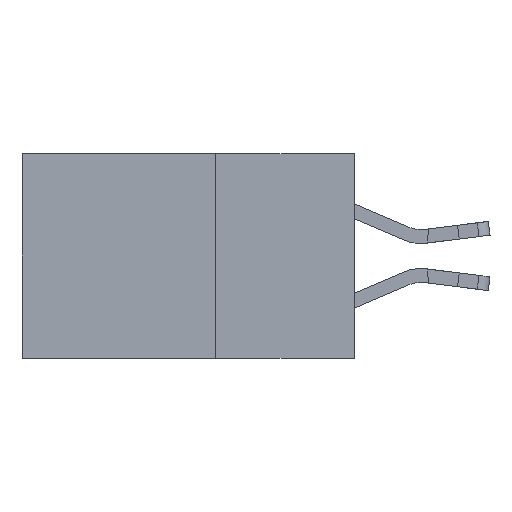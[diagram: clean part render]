
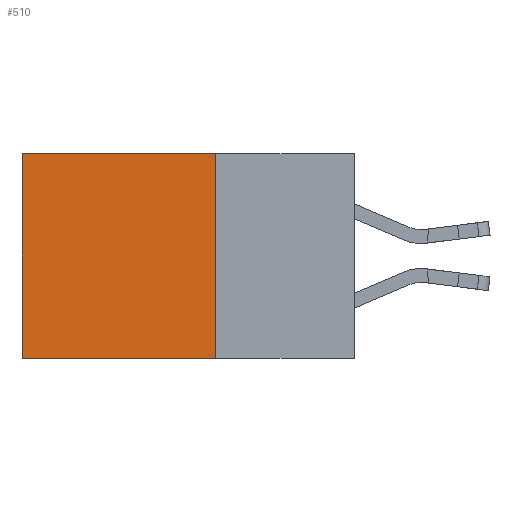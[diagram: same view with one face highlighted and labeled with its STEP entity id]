
A CAD part, left-side view. The second image highlights one B-rep face of the part: STEP entity #510.
In plain terms, the highlighted planar face has unit normal (-1, 0, 0).
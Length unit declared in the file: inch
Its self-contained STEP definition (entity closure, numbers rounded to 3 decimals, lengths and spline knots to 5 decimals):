
#156 = LINE ( 'NONE', #444, #13426 ) ;
#444 = CARTESIAN_POINT ( 'NONE',  ( 0.298, 0.6, 0. ) ) ;
#510 = ADVANCED_FACE ( 'NONE', ( #1798 ), #8470, .F. ) ;
#1036 = CARTESIAN_POINT ( 'NONE',  ( 0.298, 0.25, 0. ) ) ;
#1798 = FACE_OUTER_BOUND ( 'NONE', #5750, .T. ) ;
#1811 = LINE ( 'NONE', #9226, #8210 ) ;
#2657 = CARTESIAN_POINT ( 'NONE',  ( 0.298, 0.25, -0.37 ) ) ;
#3280 = DIRECTION ( 'NONE',  ( 0., 1., 0. ) ) ;
#3927 = ORIENTED_EDGE ( 'NONE', *, *, #4398, .F. ) ;
#4270 = ORIENTED_EDGE ( 'NONE', *, *, #12118, .T. ) ;
#4398 = EDGE_CURVE ( 'NONE', #7279, #4654, #6225, .T. ) ;
#4654 = VERTEX_POINT ( 'NONE', #10276 ) ;
#5217 = VECTOR ( 'NONE', #14128, 39.37008 ) ;
#5750 = EDGE_LOOP ( 'NONE', ( #12207, #3927, #15082, #4270 ) ) ;
#5887 = DIRECTION ( 'NONE',  ( 0., 0., -1. ) ) ;
#6090 = EDGE_CURVE ( 'NONE', #11972, #4654, #156, .T. ) ;
#6225 = LINE ( 'NONE', #8541, #9067 ) ;
#6424 = LINE ( 'NONE', #9125, #5217 ) ;
#6779 = DIRECTION ( 'NONE',  ( 0., 0., -1. ) ) ;
#7130 = DIRECTION ( 'NONE',  ( 1., 0., 0. ) ) ;
#7186 = CARTESIAN_POINT ( 'NONE',  ( 0.298, 0.25, 0. ) ) ;
#7279 = VERTEX_POINT ( 'NONE', #2657 ) ;
#8210 = VECTOR ( 'NONE', #9119, 39.37008 ) ;
#8470 = PLANE ( 'NONE',  #15882 ) ;
#8541 = CARTESIAN_POINT ( 'NONE',  ( 0.298, 0.25, -0.37 ) ) ;
#9067 = VECTOR ( 'NONE', #3280, 39.37008 ) ;
#9119 = DIRECTION ( 'NONE',  ( 0., 0., -1. ) ) ;
#9125 = CARTESIAN_POINT ( 'NONE',  ( 0.298, 0.25, 0. ) ) ;
#9226 = CARTESIAN_POINT ( 'NONE',  ( 0.298, 0.25, 0. ) ) ;
#10276 = CARTESIAN_POINT ( 'NONE',  ( 0.298, 0.6, -0.37 ) ) ;
#11183 = CARTESIAN_POINT ( 'NONE',  ( 0.298, 0.6, 0. ) ) ;
#11972 = VERTEX_POINT ( 'NONE', #11183 ) ;
#12118 = EDGE_CURVE ( 'NONE', #12897, #11972, #6424, .T. ) ;
#12207 = ORIENTED_EDGE ( 'NONE', *, *, #6090, .T. ) ;
#12897 = VERTEX_POINT ( 'NONE', #1036 ) ;
#13271 = EDGE_CURVE ( 'NONE', #12897, #7279, #1811, .T. ) ;
#13426 = VECTOR ( 'NONE', #6779, 39.37008 ) ;
#14128 = DIRECTION ( 'NONE',  ( 0., 1., 0. ) ) ;
#15082 = ORIENTED_EDGE ( 'NONE', *, *, #13271, .F. ) ;
#15882 = AXIS2_PLACEMENT_3D ( 'NONE', #7186, #7130, #5887 ) ;
